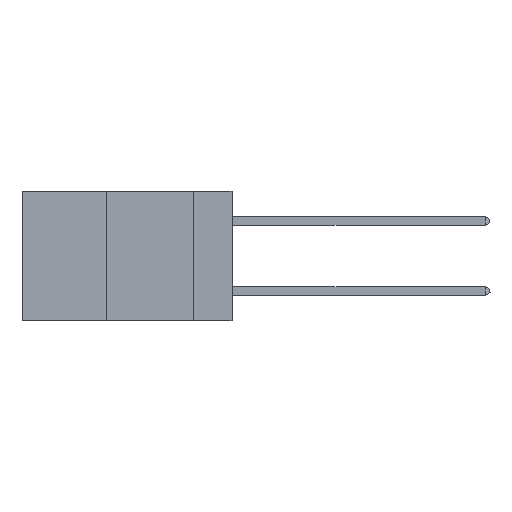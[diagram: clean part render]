
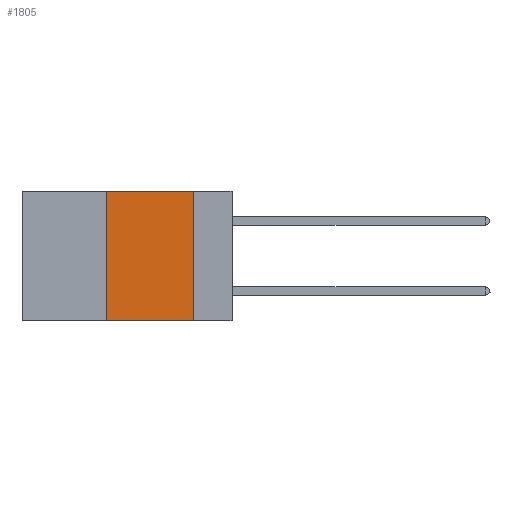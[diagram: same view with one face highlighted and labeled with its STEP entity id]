
A CAD part, left-side view. The second image highlights one B-rep face of the part: STEP entity #1805.
In plain terms, the highlighted planar face has unit normal (-1, 0, 0).
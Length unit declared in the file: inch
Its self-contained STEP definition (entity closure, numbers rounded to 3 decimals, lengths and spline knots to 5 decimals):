
#279 = PLANE ( 'NONE',  #9141 ) ;
#317 = ORIENTED_EDGE ( 'NONE', *, *, #10212, .T. ) ;
#328 = ORIENTED_EDGE ( 'NONE', *, *, #14118, .F. ) ;
#474 = VERTEX_POINT ( 'NONE', #9825 ) ;
#504 = CARTESIAN_POINT ( 'NONE',  ( 0., 0.11, 0. ) ) ;
#1129 = VECTOR ( 'NONE', #12044, 39.37008 ) ;
#1805 = ADVANCED_FACE ( 'NONE', ( #14156 ), #279, .F. ) ;
#2445 = VERTEX_POINT ( 'NONE', #9743 ) ;
#2540 = CARTESIAN_POINT ( 'NONE',  ( 0., 0.6, 0. ) ) ;
#2727 = LINE ( 'NONE', #504, #1129 ) ;
#3403 = CARTESIAN_POINT ( 'NONE',  ( 0., 0.6, -0.37 ) ) ;
#3699 = DIRECTION ( 'NONE',  ( 0., 0., -1. ) ) ;
#4500 = CARTESIAN_POINT ( 'NONE',  ( 0., 0.36, 0. ) ) ;
#4553 = EDGE_CURVE ( 'NONE', #6898, #2445, #9154, .T. ) ;
#4682 = VECTOR ( 'NONE', #13504, 39.37008 ) ;
#5378 = EDGE_CURVE ( 'NONE', #474, #6898, #9936, .T. ) ;
#5541 = VERTEX_POINT ( 'NONE', #10543 ) ;
#6282 = CARTESIAN_POINT ( 'NONE',  ( 0., 0.36, 0. ) ) ;
#6870 = CARTESIAN_POINT ( 'NONE',  ( 0., 0.6, 0. ) ) ;
#6898 = VERTEX_POINT ( 'NONE', #6282 ) ;
#8382 = VECTOR ( 'NONE', #8971, 39.37008 ) ;
#8971 = DIRECTION ( 'NONE',  ( 0., -1., 0. ) ) ;
#9052 = ORIENTED_EDGE ( 'NONE', *, *, #4553, .F. ) ;
#9141 = AXIS2_PLACEMENT_3D ( 'NONE', #2540, #10563, #3699 ) ;
#9154 = LINE ( 'NONE', #6870, #4682 ) ;
#9419 = VECTOR ( 'NONE', #11349, 39.37008 ) ;
#9743 = CARTESIAN_POINT ( 'NONE',  ( 0., 0.11, 0. ) ) ;
#9825 = CARTESIAN_POINT ( 'NONE',  ( 0., 0.36, -0.37 ) ) ;
#9936 = LINE ( 'NONE', #4500, #9419 ) ;
#10212 = EDGE_CURVE ( 'NONE', #474, #5541, #10710, .T. ) ;
#10377 = EDGE_LOOP ( 'NONE', ( #328, #9052, #13971, #317 ) ) ;
#10543 = CARTESIAN_POINT ( 'NONE',  ( 0., 0.11, -0.37 ) ) ;
#10563 = DIRECTION ( 'NONE',  ( 1., 0., 0. ) ) ;
#10710 = LINE ( 'NONE', #3403, #8382 ) ;
#11349 = DIRECTION ( 'NONE',  ( 0., 0., 1. ) ) ;
#12044 = DIRECTION ( 'NONE',  ( 0., 0., -1. ) ) ;
#13504 = DIRECTION ( 'NONE',  ( 0., -1., 0. ) ) ;
#13971 = ORIENTED_EDGE ( 'NONE', *, *, #5378, .F. ) ;
#14118 = EDGE_CURVE ( 'NONE', #2445, #5541, #2727, .T. ) ;
#14156 = FACE_OUTER_BOUND ( 'NONE', #10377, .T. ) ;
